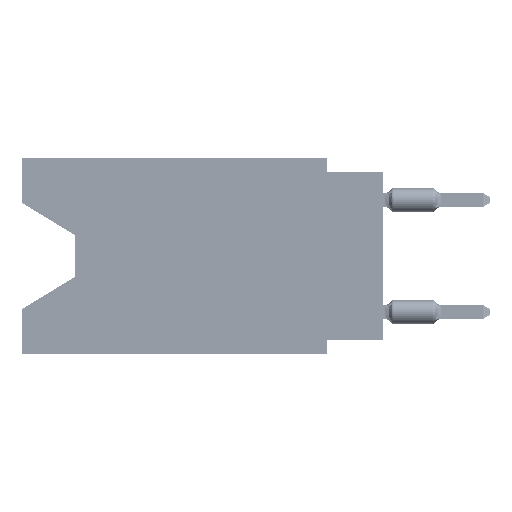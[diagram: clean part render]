
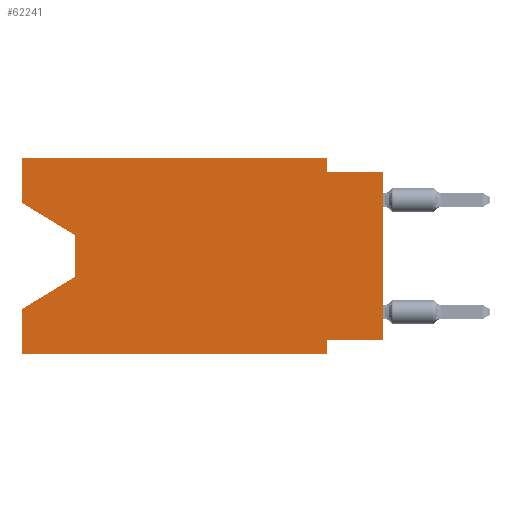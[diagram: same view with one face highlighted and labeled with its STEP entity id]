
A CAD part, left-side view. The second image highlights one B-rep face of the part: STEP entity #62241.
In plain terms, the highlighted planar face has unit normal (-1, 0, 0).
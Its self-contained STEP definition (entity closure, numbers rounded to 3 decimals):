
#1050 = ORIENTED_EDGE ( 'NONE', *, *, #23476, .T. ) ;
#1889 = LINE ( 'NONE', #25728, #23500 ) ;
#3240 = VERTEX_POINT ( 'NONE', #21291 ) ;
#3349 = ORIENTED_EDGE ( 'NONE', *, *, #51020, .T. ) ;
#3819 = EDGE_CURVE ( 'NONE', #3240, #30478, #5154, .T. ) ;
#4001 = CARTESIAN_POINT ( 'NONE',  ( 0., 2.54, -8.89 ) ) ;
#4317 = EDGE_CURVE ( 'NONE', #48822, #69958, #16568, .T. ) ;
#4385 = DIRECTION ( 'NONE',  ( 0., 0., -1. ) ) ;
#4973 = ORIENTED_EDGE ( 'NONE', *, *, #12343, .F. ) ;
#5154 = LINE ( 'NONE', #4001, #63344 ) ;
#5947 = VECTOR ( 'NONE', #58096, 1000. ) ;
#6070 = VECTOR ( 'NONE', #61817, 1000. ) ;
#7434 = ORIENTED_EDGE ( 'NONE', *, *, #18234, .F. ) ;
#8636 = LINE ( 'NONE', #50076, #6070 ) ;
#8643 = EDGE_CURVE ( 'NONE', #73345, #48822, #38088, .T. ) ;
#9252 = DIRECTION ( 'NONE',  ( 0., 0., -1. ) ) ;
#10166 = CARTESIAN_POINT ( 'NONE',  ( 0., 16.383, -2.038 ) ) ;
#10364 = LINE ( 'NONE', #11141, #20339 ) ;
#10543 = ORIENTED_EDGE ( 'NONE', *, *, #8643, .F. ) ;
#11141 = CARTESIAN_POINT ( 'NONE',  ( 0., 16.383, 0. ) ) ;
#12343 = EDGE_CURVE ( 'NONE', #67859, #3240, #25596, .T. ) ;
#12628 = CARTESIAN_POINT ( 'NONE',  ( 0., 16.383, 0. ) ) ;
#13382 = CARTESIAN_POINT ( 'NONE',  ( 0., 13.97, -5.385 ) ) ;
#14718 = VECTOR ( 'NONE', #40967, 1000. ) ;
#14850 = VERTEX_POINT ( 'NONE', #41958 ) ;
#16410 = LINE ( 'NONE', #10166, #61921 ) ;
#16568 = LINE ( 'NONE', #28289, #54686 ) ;
#17030 = CARTESIAN_POINT ( 'NONE',  ( 0., 0., 0. ) ) ;
#17520 = DIRECTION ( 'NONE',  ( 0., 0., -1. ) ) ;
#18234 = EDGE_CURVE ( 'NONE', #52218, #14850, #20388, .T. ) ;
#20059 = EDGE_CURVE ( 'NONE', #31845, #55723, #39808, .T. ) ;
#20247 = EDGE_CURVE ( 'NONE', #35838, #73345, #10364, .T. ) ;
#20339 = VECTOR ( 'NONE', #64675, 1000. ) ;
#20388 = LINE ( 'NONE', #44230, #30101 ) ;
#20522 = VECTOR ( 'NONE', #40868, 1000. ) ;
#21291 = CARTESIAN_POINT ( 'NONE',  ( 0., 2.54, -8.255 ) ) ;
#22713 = ORIENTED_EDGE ( 'NONE', *, *, #4317, .F. ) ;
#22937 = CARTESIAN_POINT ( 'NONE',  ( 0., 13.97, -3.505 ) ) ;
#23381 = CARTESIAN_POINT ( 'NONE',  ( 0., 13.97, -3.505 ) ) ;
#23476 = EDGE_CURVE ( 'NONE', #67859, #71003, #70551, .T. ) ;
#23500 = VECTOR ( 'NONE', #49580, 1000. ) ;
#25207 = CARTESIAN_POINT ( 'NONE',  ( 0., 0., -8.255 ) ) ;
#25596 = LINE ( 'NONE', #25207, #14718 ) ;
#25728 = CARTESIAN_POINT ( 'NONE',  ( 0., 16.383, -8.89 ) ) ;
#26384 = CARTESIAN_POINT ( 'NONE',  ( 0., 2.54, -8.89 ) ) ;
#26394 = CARTESIAN_POINT ( 'NONE',  ( 0., 2.54, 0. ) ) ;
#27908 = ORIENTED_EDGE ( 'NONE', *, *, #20059, .T. ) ;
#28289 = CARTESIAN_POINT ( 'NONE',  ( 0., 2.54, 0. ) ) ;
#30101 = VECTOR ( 'NONE', #57490, 1000. ) ;
#30478 = VERTEX_POINT ( 'NONE', #26384 ) ;
#31557 = PLANE ( 'NONE',  #58257 ) ;
#31845 = VERTEX_POINT ( 'NONE', #22937 ) ;
#32198 = CARTESIAN_POINT ( 'NONE',  ( 0., 16.383, -2.038 ) ) ;
#32619 = CARTESIAN_POINT ( 'NONE',  ( 0., 16.383, 0. ) ) ;
#33139 = VECTOR ( 'NONE', #44339, 1000. ) ;
#34634 = CARTESIAN_POINT ( 'NONE',  ( 0., 0., -0.635 ) ) ;
#35838 = VERTEX_POINT ( 'NONE', #32198 ) ;
#38088 = LINE ( 'NONE', #32619, #33139 ) ;
#38951 = FACE_OUTER_BOUND ( 'NONE', #65963, .T. ) ;
#39808 = LINE ( 'NONE', #23381, #65243 ) ;
#40868 = DIRECTION ( 'NONE',  ( 0., 0., 1. ) ) ;
#40884 = LINE ( 'NONE', #34634, #5947 ) ;
#40967 = DIRECTION ( 'NONE',  ( 0., 1., 0. ) ) ;
#41958 = CARTESIAN_POINT ( 'NONE',  ( 0., 16.383, -6.852 ) ) ;
#43784 = EDGE_CURVE ( 'NONE', #69958, #71003, #40884, .T. ) ;
#44230 = CARTESIAN_POINT ( 'NONE',  ( 0., 16.383, 0. ) ) ;
#44339 = DIRECTION ( 'NONE',  ( 0., -1., 0. ) ) ;
#45879 = DIRECTION ( 'NONE',  ( 0., 0., -1. ) ) ;
#48114 = CARTESIAN_POINT ( 'NONE',  ( 0., 16.383, -8.89 ) ) ;
#48822 = VERTEX_POINT ( 'NONE', #26394 ) ;
#49580 = DIRECTION ( 'NONE',  ( 0., -1., 0. ) ) ;
#50076 = CARTESIAN_POINT ( 'NONE',  ( 0., 13.97, -5.385 ) ) ;
#50271 = ORIENTED_EDGE ( 'NONE', *, *, #65790, .T. ) ;
#51020 = EDGE_CURVE ( 'NONE', #35838, #31845, #16410, .T. ) ;
#52218 = VERTEX_POINT ( 'NONE', #48114 ) ;
#52975 = EDGE_CURVE ( 'NONE', #55723, #14850, #8636, .T. ) ;
#53157 = ORIENTED_EDGE ( 'NONE', *, *, #3819, .F. ) ;
#54686 = VECTOR ( 'NONE', #45879, 1000. ) ;
#55402 = CARTESIAN_POINT ( 'NONE',  ( 0., 16.383, 0. ) ) ;
#55723 = VERTEX_POINT ( 'NONE', #13382 ) ;
#55948 = CARTESIAN_POINT ( 'NONE',  ( 0., 2.54, -0.635 ) ) ;
#57095 = ORIENTED_EDGE ( 'NONE', *, *, #43784, .F. ) ;
#57490 = DIRECTION ( 'NONE',  ( 0., 0., 1. ) ) ;
#58096 = DIRECTION ( 'NONE',  ( 0., -1., 0. ) ) ;
#58257 = AXIS2_PLACEMENT_3D ( 'NONE', #55402, #62812, #9252 ) ;
#61050 = CARTESIAN_POINT ( 'NONE',  ( 0., 0., -0.635 ) ) ;
#61817 = DIRECTION ( 'NONE',  ( 0., 0.855, -0.519 ) ) ;
#61921 = VECTOR ( 'NONE', #68788, 1000. ) ;
#62241 = ADVANCED_FACE ( 'NONE', ( #38951 ), #31557, .F. ) ;
#62812 = DIRECTION ( 'NONE',  ( 1., 0., 0. ) ) ;
#63344 = VECTOR ( 'NONE', #4385, 1000. ) ;
#64675 = DIRECTION ( 'NONE',  ( 0., 0., 1. ) ) ;
#65243 = VECTOR ( 'NONE', #17520, 1000. ) ;
#65790 = EDGE_CURVE ( 'NONE', #52218, #30478, #1889, .T. ) ;
#65963 = EDGE_LOOP ( 'NONE', ( #3349, #27908, #70883, #7434, #50271, #53157, #4973, #1050, #57095, #22713, #10543, #76234 ) ) ;
#67378 = CARTESIAN_POINT ( 'NONE',  ( 0., 0., -8.255 ) ) ;
#67859 = VERTEX_POINT ( 'NONE', #67378 ) ;
#68788 = DIRECTION ( 'NONE',  ( 0., -0.855, -0.519 ) ) ;
#69958 = VERTEX_POINT ( 'NONE', #55948 ) ;
#70551 = LINE ( 'NONE', #17030, #20522 ) ;
#70883 = ORIENTED_EDGE ( 'NONE', *, *, #52975, .T. ) ;
#71003 = VERTEX_POINT ( 'NONE', #61050 ) ;
#73345 = VERTEX_POINT ( 'NONE', #12628 ) ;
#76234 = ORIENTED_EDGE ( 'NONE', *, *, #20247, .F. ) ;
